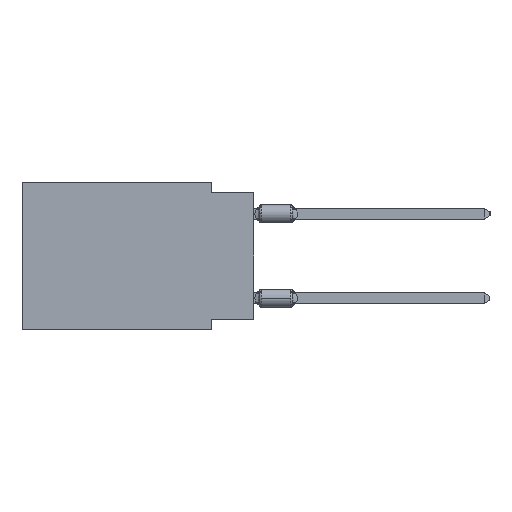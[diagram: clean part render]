
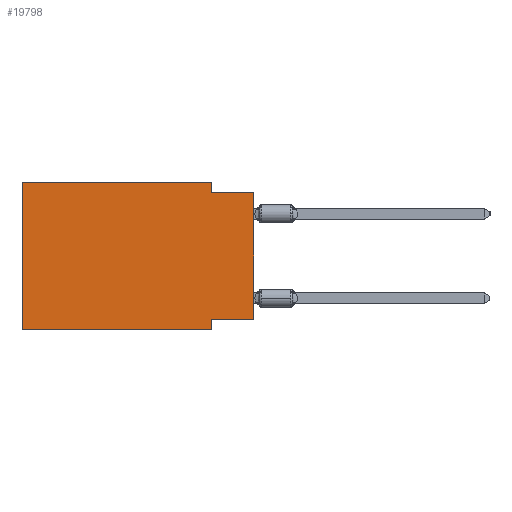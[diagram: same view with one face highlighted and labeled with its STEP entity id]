
A CAD part, left-side view. The second image highlights one B-rep face of the part: STEP entity #19798.
In plain terms, the highlighted planar face has unit normal (-1, 0, 0).
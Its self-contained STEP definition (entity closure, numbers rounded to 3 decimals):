
#102 = CARTESIAN_POINT ( 'NONE',  ( 0., 2.54, -8.89 ) ) ;
#300 = DIRECTION ( 'NONE',  ( 0., 0., 1. ) ) ;
#1130 = VERTEX_POINT ( 'NONE', #31472 ) ;
#1460 = EDGE_CURVE ( 'NONE', #27517, #27989, #31782, .T. ) ;
#2493 = ORIENTED_EDGE ( 'NONE', *, *, #1460, .F. ) ;
#2624 = LINE ( 'NONE', #7549, #27436 ) ;
#3070 = PLANE ( 'NONE',  #15206 ) ;
#3800 = EDGE_CURVE ( 'NONE', #28442, #1130, #31277, .T. ) ;
#3986 = DIRECTION ( 'NONE',  ( 0., -1., 0. ) ) ;
#4162 = LINE ( 'NONE', #18322, #13407 ) ;
#4604 = VERTEX_POINT ( 'NONE', #12420 ) ;
#4889 = DIRECTION ( 'NONE',  ( 0., 0., -1. ) ) ;
#5540 = EDGE_CURVE ( 'NONE', #26283, #28442, #13416, .T. ) ;
#5987 = DIRECTION ( 'NONE',  ( 0., -1., 0. ) ) ;
#7375 = EDGE_CURVE ( 'NONE', #36975, #4604, #4162, .T. ) ;
#7549 = CARTESIAN_POINT ( 'NONE',  ( 0., 2.54, 0. ) ) ;
#8832 = CARTESIAN_POINT ( 'NONE',  ( 0., 13.97, -8.89 ) ) ;
#9391 = DIRECTION ( 'NONE',  ( 0., -1., 0. ) ) ;
#10452 = CARTESIAN_POINT ( 'NONE',  ( 0., 2.54, -8.89 ) ) ;
#10594 = CARTESIAN_POINT ( 'NONE',  ( 0., 13.97, 0. ) ) ;
#11105 = CARTESIAN_POINT ( 'NONE',  ( 0., 13.97, 0. ) ) ;
#11236 = DIRECTION ( 'NONE',  ( 0., 0., -1. ) ) ;
#11257 = VERTEX_POINT ( 'NONE', #32320 ) ;
#11555 = VECTOR ( 'NONE', #300, 1000. ) ;
#11682 = VECTOR ( 'NONE', #18140, 1000. ) ;
#12420 = CARTESIAN_POINT ( 'NONE',  ( 0., 0., -0.635 ) ) ;
#12841 = ORIENTED_EDGE ( 'NONE', *, *, #34292, .F. ) ;
#13407 = VECTOR ( 'NONE', #3986, 1000. ) ;
#13416 = LINE ( 'NONE', #10594, #15724 ) ;
#14770 = DIRECTION ( 'NONE',  ( 1., 0., 0. ) ) ;
#15206 = AXIS2_PLACEMENT_3D ( 'NONE', #37220, #14770, #25723 ) ;
#15543 = EDGE_CURVE ( 'NONE', #26283, #27989, #23919, .T. ) ;
#15724 = VECTOR ( 'NONE', #34141, 1000. ) ;
#16779 = ORIENTED_EDGE ( 'NONE', *, *, #7375, .F. ) ;
#16853 = FACE_OUTER_BOUND ( 'NONE', #28250, .T. ) ;
#17367 = CARTESIAN_POINT ( 'NONE',  ( 0., 2.54, -0.635 ) ) ;
#18140 = DIRECTION ( 'NONE',  ( 0., 1., 0. ) ) ;
#18322 = CARTESIAN_POINT ( 'NONE',  ( 0., 0., -0.635 ) ) ;
#19597 = EDGE_CURVE ( 'NONE', #11257, #4604, #26140, .T. ) ;
#19634 = CARTESIAN_POINT ( 'NONE',  ( 0., 13.97, 0. ) ) ;
#19798 = ADVANCED_FACE ( 'NONE', ( #16853 ), #3070, .F. ) ;
#22589 = ORIENTED_EDGE ( 'NONE', *, *, #19597, .T. ) ;
#22737 = VECTOR ( 'NONE', #9391, 1000. ) ;
#23919 = LINE ( 'NONE', #8832, #22737 ) ;
#25143 = ORIENTED_EDGE ( 'NONE', *, *, #5540, .F. ) ;
#25723 = DIRECTION ( 'NONE',  ( 0., 0., -1. ) ) ;
#26140 = LINE ( 'NONE', #28786, #11555 ) ;
#26283 = VERTEX_POINT ( 'NONE', #32365 ) ;
#27436 = VECTOR ( 'NONE', #4889, 1000. ) ;
#27517 = VERTEX_POINT ( 'NONE', #35774 ) ;
#27989 = VERTEX_POINT ( 'NONE', #10452 ) ;
#28250 = EDGE_LOOP ( 'NONE', ( #22589, #16779, #12841, #30156, #25143, #28752, #2493, #30321 ) ) ;
#28274 = EDGE_CURVE ( 'NONE', #11257, #27517, #29659, .T. ) ;
#28442 = VERTEX_POINT ( 'NONE', #19634 ) ;
#28730 = VECTOR ( 'NONE', #5987, 1000. ) ;
#28752 = ORIENTED_EDGE ( 'NONE', *, *, #15543, .T. ) ;
#28786 = CARTESIAN_POINT ( 'NONE',  ( 0., 0., 0. ) ) ;
#29510 = VECTOR ( 'NONE', #11236, 1000. ) ;
#29659 = LINE ( 'NONE', #33033, #11682 ) ;
#30156 = ORIENTED_EDGE ( 'NONE', *, *, #3800, .F. ) ;
#30321 = ORIENTED_EDGE ( 'NONE', *, *, #28274, .F. ) ;
#31277 = LINE ( 'NONE', #11105, #28730 ) ;
#31472 = CARTESIAN_POINT ( 'NONE',  ( 0., 2.54, 0. ) ) ;
#31782 = LINE ( 'NONE', #102, #29510 ) ;
#32320 = CARTESIAN_POINT ( 'NONE',  ( 0., 0., -8.255 ) ) ;
#32365 = CARTESIAN_POINT ( 'NONE',  ( 0., 13.97, -8.89 ) ) ;
#33033 = CARTESIAN_POINT ( 'NONE',  ( 0., 0., -8.255 ) ) ;
#34141 = DIRECTION ( 'NONE',  ( 0., 0., 1. ) ) ;
#34292 = EDGE_CURVE ( 'NONE', #1130, #36975, #2624, .T. ) ;
#35774 = CARTESIAN_POINT ( 'NONE',  ( 0., 2.54, -8.255 ) ) ;
#36975 = VERTEX_POINT ( 'NONE', #17367 ) ;
#37220 = CARTESIAN_POINT ( 'NONE',  ( 0., 13.97, 0. ) ) ;
